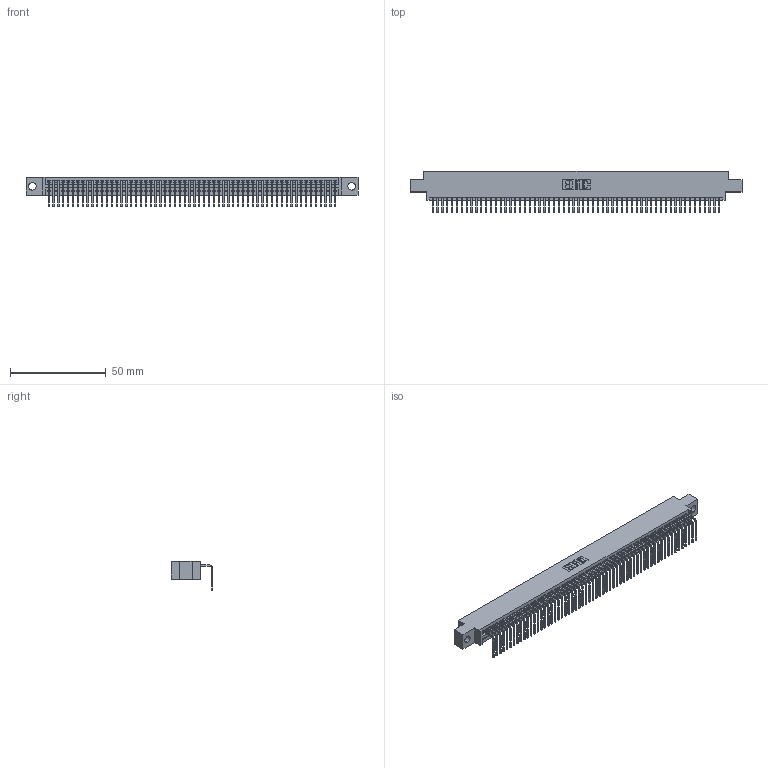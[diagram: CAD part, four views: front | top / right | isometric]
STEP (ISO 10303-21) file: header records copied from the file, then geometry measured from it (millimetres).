
FILE_DESCRIPTION (( 'STEP AP203' ), '1' );
FILE_NAME ('395-060-558-604.STEP', '2021-06-11T19:41:38', ( '' ), ( '' ), 'SwSTEP 2.0', 'SolidWorks 2020', '' );
FILE_SCHEMA (( 'CONFIG_CONTROL_DESIGN' ));
Length unit declared in the file: inch
Products named in the file (3): 345-292-001_558 Tail - 2; 345 Part_0.170 Offset - 0.156 Dia-TI; 395-060-558-604
Assembly tree (61 placements, depth 2):
  395-060-558-604
    345 Part_0.170 Offset - 0.156 Dia-TI
    345-292-001_558 Tail - 2  x60
Bounding box: 173.61 x 21.83 x 15.37 mm (x, y, z)
Volume: 16617.6 mm3; surface area: 23471.6 mm2
Topology: 61 solids, 61 shells, 3744 faces, 11309 edges, 7458 vertices
Faces by surface type: plane 2618, cylinder 1126
Entity records: 43369 total; most frequent: CARTESIAN_POINT 7522, ORIENTED_EDGE 7514, DIRECTION 6541, EDGE_CURVE 3757, VECTOR 3385, LINE 3385, VERTEX_POINT 2502, AXIS2_PLACEMENT_3D 1578
